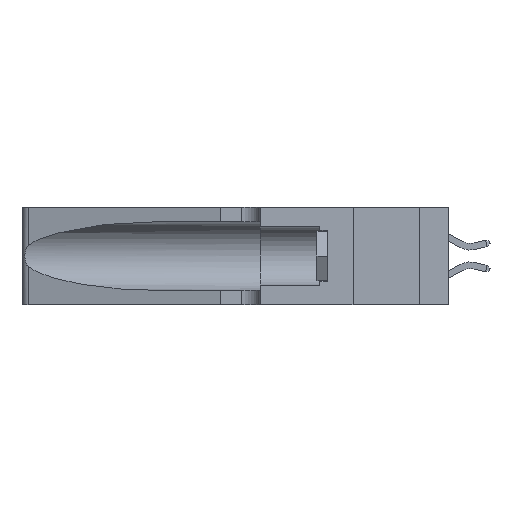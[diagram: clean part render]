
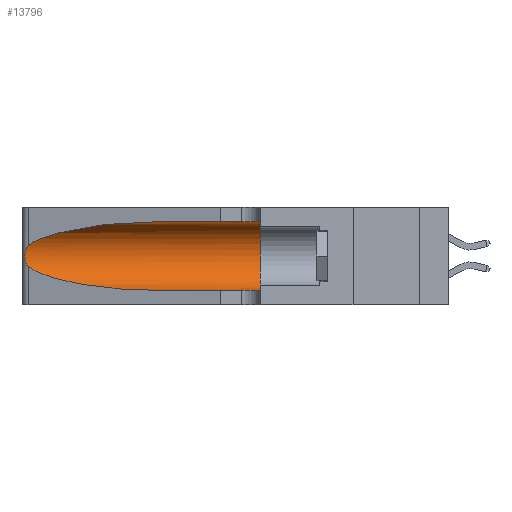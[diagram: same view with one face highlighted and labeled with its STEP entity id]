
A CAD part, left-side view. The second image highlights one B-rep face of the part: STEP entity #13796.
In plain terms, the highlighted cylindrical face has radius 3.308 mm (diameter 6.617 mm), a partial arc.
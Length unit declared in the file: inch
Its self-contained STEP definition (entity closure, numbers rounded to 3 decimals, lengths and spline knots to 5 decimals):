
#361 = CARTESIAN_POINT ( 'NONE',  ( 0.25639, 1.23184, 0.21858 ) ) ;
#1506 = CARTESIAN_POINT ( 'NONE',  ( 0.1305, 0.72297, 0.05475 ) ) ;
#1610 = CARTESIAN_POINT ( 'NONE',  ( 0.2373, 1.15595, 0.08982 ) ) ;
#2491 = CARTESIAN_POINT ( 'NONE',  ( 0.25487, 1.22718, 0.22369 ) ) ;
#2739 = CARTESIAN_POINT ( 'NONE',  ( 0.25854, 1.2359, 0.20912 ) ) ;
#2768 = VERTEX_POINT ( 'NONE', #15981 ) ;
#2975 = CARTESIAN_POINT ( 'NONE',  ( 0.25487, 1.22718, 0.14631 ) ) ;
#3694 = EDGE_CURVE ( 'NONE', #2768, #19446, #12977, .T. ) ;
#3984 = CARTESIAN_POINT ( 'NONE',  ( 0.1305, 0.72297, 0.05475 ) ) ;
#4258 = B_SPLINE_CURVE_WITH_KNOTS ( 'NONE', 3,
 ( #7404, #21135, #361, #16714, #2739, #18984, #5121, #21230, #7502, #23456, #9873, #25711, #12180, #27918 ),
 .UNSPECIFIED., .F., .F.,
 ( 4, 2, 2, 2, 2, 2, 4 ),
 ( 0., 0.00027, 0.00053, 0.00107, 0.0016, 0.00187, 0.00214 ),
 .UNSPECIFIED. ) ;
#4564 = CARTESIAN_POINT ( 'NONE',  ( 0.1305, 1.61858, 0.185 ) ) ;
#4635 = ORIENTED_EDGE ( 'NONE', *, *, #3694, .F. ) ;
#5121 = CARTESIAN_POINT ( 'NONE',  ( 0.26075, 1.23896, 0.19203 ) ) ;
#6134 = VERTEX_POINT ( 'NONE', #19324 ) ;
#6429 = CARTESIAN_POINT ( 'NONE',  ( 0.1305, 0.35, 0.185 ) ) ;
#7404 = CARTESIAN_POINT ( 'NONE',  ( 0.25487, 1.22718, 0.22369 ) ) ;
#7502 = CARTESIAN_POINT ( 'NONE',  ( 0.26017, 1.23833, 0.17102 ) ) ;
#7937 = CYLINDRICAL_SURFACE ( 'NONE', #8393, 0.13025 ) ;
#8373 = CARTESIAN_POINT ( 'NONE',  ( 0.1305, 1.61858, 0.05475 ) ) ;
#8393 = AXIS2_PLACEMENT_3D ( 'NONE', #4564, #22946, #11645 ) ;
#8566 = EDGE_CURVE ( 'NONE', #19061, #19309, #29088, .T. ) ;
#8787 = DIRECTION ( 'NONE',  ( 0., 0., 1. ) ) ;
#8981 = LINE ( 'NONE', #13492, #16580 ) ;
#9873 = CARTESIAN_POINT ( 'NONE',  ( 0.25789, 1.23486, 0.15765 ) ) ;
#9890 = ORIENTED_EDGE ( 'NONE', *, *, #20470, .T. ) ;
#10401 =( BOUNDED_CURVE ( )  B_SPLINE_CURVE ( 3, ( #25370, #18644, #16469, #2491 ),
 .UNSPECIFIED., .F., .F. ) 
 B_SPLINE_CURVE_WITH_KNOTS ( ( 4, 4 ),
 ( 1.5708, 2.84003 ),
 .UNSPECIFIED. ) 
 CURVE ( )  GEOMETRIC_REPRESENTATION_ITEM ( )  RATIONAL_B_SPLINE_CURVE ( ( 1., 0.87, 0.87, 1. ) ) 
 REPRESENTATION_ITEM ( '' )  );
#10711 = DIRECTION ( 'NONE',  ( 0., -1., 0. ) ) ;
#11645 = DIRECTION ( 'NONE',  ( 0., 0., -1. ) ) ;
#12180 = CARTESIAN_POINT ( 'NONE',  ( 0.25555, 1.22993, 0.14849 ) ) ;
#12724 = EDGE_CURVE ( 'NONE', #20094, #6134, #10401, .T. ) ;
#12977 = CIRCLE ( 'NONE', #28494, 0.13025 ) ;
#13492 = CARTESIAN_POINT ( 'NONE',  ( 0.1305, 1.61858, 0.31525 ) ) ;
#13796 = ADVANCED_FACE ( 'NONE', ( #14865 ), #7937, .F. ) ;
#14865 = FACE_OUTER_BOUND ( 'NONE', #21467, .T. ) ;
#15600 = EDGE_CURVE ( 'NONE', #20094, #2768, #8981, .T. ) ;
#15805 = DIRECTION ( 'NONE',  ( 0., -1., 0. ) ) ;
#15862 = VECTOR ( 'NONE', #10711, 39.37008 ) ;
#15907 = ORIENTED_EDGE ( 'NONE', *, *, #15600, .F. ) ;
#15981 = CARTESIAN_POINT ( 'NONE',  ( 0.1305, 0.35, 0.31525 ) ) ;
#16298 = CARTESIAN_POINT ( 'NONE',  ( 0.1305, 0.72297, 0.31525 ) ) ;
#16469 = CARTESIAN_POINT ( 'NONE',  ( 0.2373, 1.15595, 0.28018 ) ) ;
#16580 = VECTOR ( 'NONE', #15805, 39.37008 ) ;
#16714 = CARTESIAN_POINT ( 'NONE',  ( 0.25787, 1.23484, 0.2124 ) ) ;
#17293 = LINE ( 'NONE', #8373, #15862 ) ;
#17923 = CARTESIAN_POINT ( 'NONE',  ( 0.18966, 0.96281, 0.05475 ) ) ;
#18644 = CARTESIAN_POINT ( 'NONE',  ( 0.18966, 0.96281, 0.31525 ) ) ;
#18984 = CARTESIAN_POINT ( 'NONE',  ( 0.26018, 1.23835, 0.19895 ) ) ;
#19061 = VERTEX_POINT ( 'NONE', #2975 ) ;
#19309 = VERTEX_POINT ( 'NONE', #1506 ) ;
#19324 = CARTESIAN_POINT ( 'NONE',  ( 0.25487, 1.22718, 0.22369 ) ) ;
#19446 = VERTEX_POINT ( 'NONE', #24914 ) ;
#20094 = VERTEX_POINT ( 'NONE', #16298 ) ;
#20156 = ORIENTED_EDGE ( 'NONE', *, *, #25205, .T. ) ;
#20470 = EDGE_CURVE ( 'NONE', #19309, #19446, #17293, .T. ) ;
#21135 = CARTESIAN_POINT ( 'NONE',  ( 0.25555, 1.22994, 0.2215 ) ) ;
#21230 = CARTESIAN_POINT ( 'NONE',  ( 0.26075, 1.23896, 0.178 ) ) ;
#21467 = EDGE_LOOP ( 'NONE', ( #25575, #20156, #26352, #9890, #4635, #15907 ) ) ;
#22418 = DIRECTION ( 'NONE',  ( 0., 1., 0. ) ) ;
#22946 = DIRECTION ( 'NONE',  ( 0., -1., 0. ) ) ;
#23456 = CARTESIAN_POINT ( 'NONE',  ( 0.25856, 1.23593, 0.16098 ) ) ;
#24914 = CARTESIAN_POINT ( 'NONE',  ( 0.1305, 0.35, 0.05475 ) ) ;
#25205 = EDGE_CURVE ( 'NONE', #6134, #19061, #4258, .T. ) ;
#25370 = CARTESIAN_POINT ( 'NONE',  ( 0.1305, 0.72297, 0.31525 ) ) ;
#25575 = ORIENTED_EDGE ( 'NONE', *, *, #12724, .T. ) ;
#25711 = CARTESIAN_POINT ( 'NONE',  ( 0.25639, 1.23186, 0.15144 ) ) ;
#26352 = ORIENTED_EDGE ( 'NONE', *, *, #8566, .T. ) ;
#27918 = CARTESIAN_POINT ( 'NONE',  ( 0.25487, 1.22718, 0.14631 ) ) ;
#28494 = AXIS2_PLACEMENT_3D ( 'NONE', #6429, #22418, #8787 ) ;
#28916 = CARTESIAN_POINT ( 'NONE',  ( 0.25487, 1.22718, 0.14631 ) ) ;
#29088 =( BOUNDED_CURVE ( )  B_SPLINE_CURVE ( 3, ( #28916, #1610, #17923, #3984 ),
 .UNSPECIFIED., .F., .F. ) 
 B_SPLINE_CURVE_WITH_KNOTS ( ( 4, 4 ),
 ( 3.44316, 4.71239 ),
 .UNSPECIFIED. ) 
 CURVE ( )  GEOMETRIC_REPRESENTATION_ITEM ( )  RATIONAL_B_SPLINE_CURVE ( ( 1., 0.87, 0.87, 1. ) ) 
 REPRESENTATION_ITEM ( '' )  );
